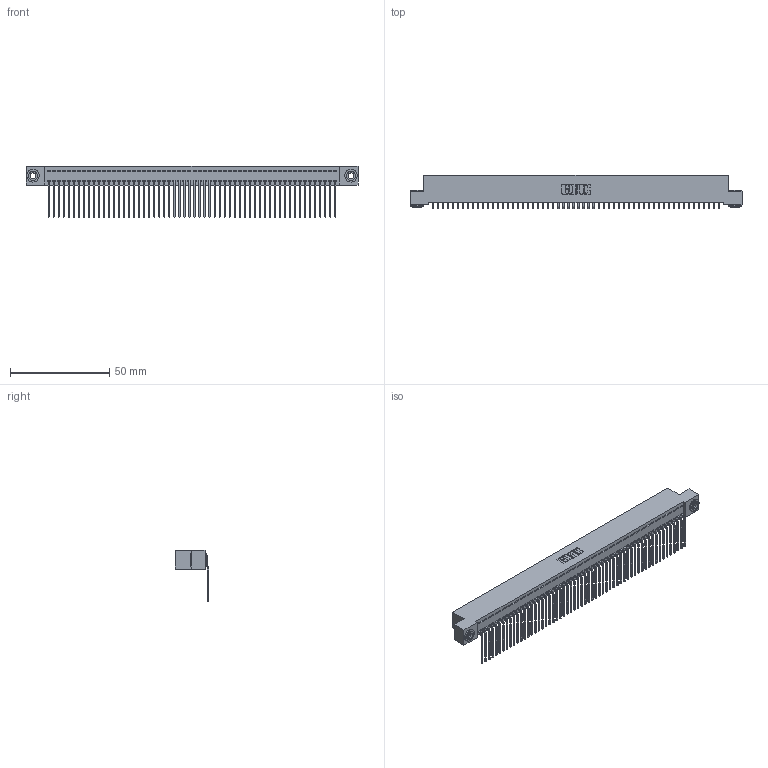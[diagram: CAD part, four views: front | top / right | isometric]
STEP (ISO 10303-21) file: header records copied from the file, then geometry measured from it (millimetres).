
FILE_DESCRIPTION (( 'STEP AP203' ), '1' );
FILE_NAME ('392-058-559-103.STEP', '2019-10-08T17:02:23', ( '' ), ( '' ), 'SwSTEP 2.0', 'SolidWorks 2016', '' );
FILE_SCHEMA (( 'CONFIG_CONTROL_DESIGN' ));
Length unit declared in the file: inch
Products named in the file (4): 342 Part_.156 TH; 345-292-001_558 559 Tail - 1; 342-250-002_345-250-002-102; 392-058-559-103
Assembly tree (61 placements, depth 2):
  392-058-559-103
    342 Part_.156 TH
    345-292-001_558 559 Tail - 1  x58
    342-250-002_345-250-002-102  x2
Bounding box: 167.64 x 16.83 x 25.78 mm (x, y, z)
Volume: 14973.7 mm3; surface area: 23610.5 mm2
Topology: 61 solids, 61 shells, 3628 faces, 10931 edges, 7206 vertices
Faces by surface type: plane 2628, cylinder 992, cone 8
Entity records: 33990 total; most frequent: CARTESIAN_POINT 5839, ORIENTED_EDGE 5826, DIRECTION 4927, EDGE_CURVE 2913, LINE 2761, VECTOR 2761, VERTEX_POINT 1938, AXIS2_PLACEMENT_3D 1083
